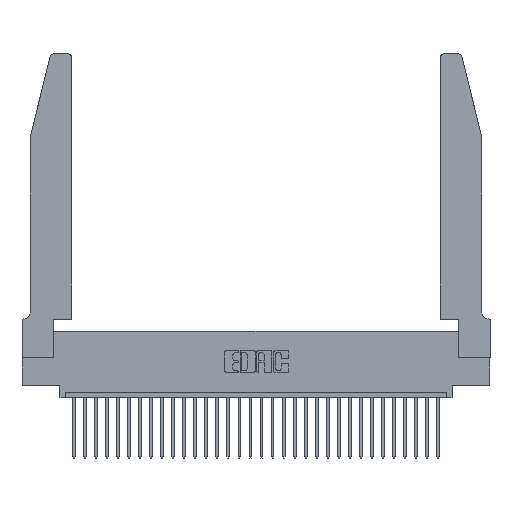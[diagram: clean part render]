
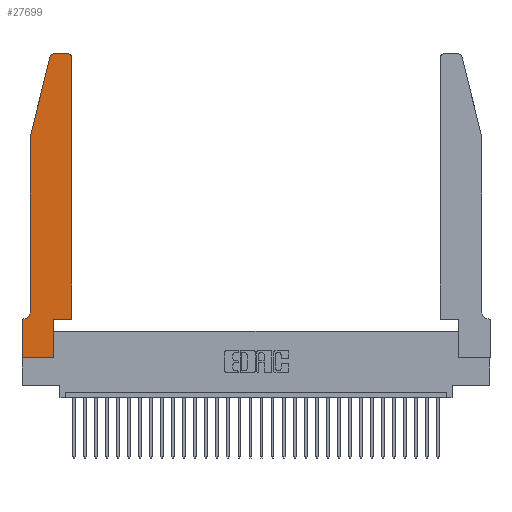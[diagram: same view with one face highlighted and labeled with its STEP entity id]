
A CAD part, top view. The second image highlights one B-rep face of the part: STEP entity #27699.
In plain terms, the highlighted planar face has unit normal (0, 0, 1).
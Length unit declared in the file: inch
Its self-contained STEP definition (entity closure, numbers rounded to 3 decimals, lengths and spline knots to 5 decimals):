
#193 = ORIENTED_EDGE ( 'NONE', *, *, #10194, .T. ) ;
#328 = CARTESIAN_POINT ( 'NONE',  ( 0.2605, 2.75, 0.37 ) ) ;
#443 = VERTEX_POINT ( 'NONE', #21732 ) ;
#835 = CARTESIAN_POINT ( 'NONE',  ( 0.0755, 2., 0.37 ) ) ;
#1008 = EDGE_CURVE ( 'NONE', #13821, #19649, #5356, .T. ) ;
#1247 = DIRECTION ( 'NONE',  ( 0., 0., 1. ) ) ;
#1374 = DIRECTION ( 'NONE',  ( 1., 0., 0. ) ) ;
#1831 = EDGE_CURVE ( 'NONE', #30188, #12874, #20572, .T. ) ;
#1934 = LINE ( 'NONE', #30293, #8049 ) ;
#1952 = CARTESIAN_POINT ( 'NONE',  ( 0.0055, 0.42, 0.37 ) ) ;
#2364 = LINE ( 'NONE', #5169, #30984 ) ;
#3104 = CARTESIAN_POINT ( 'NONE',  ( 0.0755, 0.35, 0.37 ) ) ;
#3563 = EDGE_CURVE ( 'NONE', #7966, #5126, #23149, .T. ) ;
#5004 = ORIENTED_EDGE ( 'NONE', *, *, #28620, .T. ) ;
#5009 = CARTESIAN_POINT ( 'NONE',  ( 0.0055, 0.35, 0.37 ) ) ;
#5010 = VERTEX_POINT ( 'NONE', #17199 ) ;
#5126 = VERTEX_POINT ( 'NONE', #21853 ) ;
#5169 = CARTESIAN_POINT ( 'NONE',  ( 0., 0., 0.37 ) ) ;
#5356 = CIRCLE ( 'NONE', #21744, 0.03 ) ;
#5388 = VERTEX_POINT ( 'NONE', #5009 ) ;
#5999 = EDGE_CURVE ( 'NONE', #15952, #17860, #22972, .T. ) ;
#6117 = CARTESIAN_POINT ( 'NONE',  ( 0.4505, 2.72, 0.37 ) ) ;
#6141 = DIRECTION ( 'NONE',  ( 0., 0., 1. ) ) ;
#6283 = CARTESIAN_POINT ( 'NONE',  ( 0., 0.35, 0.37 ) ) ;
#6318 = VECTOR ( 'NONE', #25117, 39.37008 ) ;
#7792 = DIRECTION ( 'NONE',  ( -1., 0., 0. ) ) ;
#7966 = VERTEX_POINT ( 'NONE', #12663 ) ;
#8049 = VECTOR ( 'NONE', #19471, 39.37008 ) ;
#8314 = DIRECTION ( 'NONE',  ( 0., 1., 0. ) ) ;
#9087 = CARTESIAN_POINT ( 'NONE',  ( 0.0755, 0.42, 0.37 ) ) ;
#9263 = DIRECTION ( 'NONE',  ( 1., 0., 0. ) ) ;
#10145 = CARTESIAN_POINT ( 'NONE',  ( 0.2865, 0.35, 0.37 ) ) ;
#10194 = EDGE_CURVE ( 'NONE', #5388, #23046, #20804, .T. ) ;
#10940 = ORIENTED_EDGE ( 'NONE', *, *, #12005, .T. ) ;
#11114 = DIRECTION ( 'NONE',  ( 0., -1., 0. ) ) ;
#11465 = VECTOR ( 'NONE', #12480, 39.37008 ) ;
#11828 = DIRECTION ( 'NONE',  ( 0., 0., 1. ) ) ;
#12005 = EDGE_CURVE ( 'NONE', #17860, #13821, #12695, .T. ) ;
#12480 = DIRECTION ( 'NONE',  ( 1., 0., 0. ) ) ;
#12663 = CARTESIAN_POINT ( 'NONE',  ( 0.2865, 0.35, 0.37 ) ) ;
#12695 = LINE ( 'NONE', #328, #15411 ) ;
#12874 = VERTEX_POINT ( 'NONE', #9087 ) ;
#13300 = DIRECTION ( 'NONE',  ( 1., 0., 0. ) ) ;
#13702 = AXIS2_PLACEMENT_3D ( 'NONE', #6283, #1247, #18309 ) ;
#13821 = VERTEX_POINT ( 'NONE', #20602 ) ;
#14493 = ORIENTED_EDGE ( 'NONE', *, *, #25346, .T. ) ;
#14534 = LINE ( 'NONE', #27191, #11465 ) ;
#14662 = ORIENTED_EDGE ( 'NONE', *, *, #5999, .T. ) ;
#15411 = VECTOR ( 'NONE', #7792, 39.37008 ) ;
#15952 = VERTEX_POINT ( 'NONE', #6117 ) ;
#16477 = ORIENTED_EDGE ( 'NONE', *, *, #1008, .T. ) ;
#16829 = CARTESIAN_POINT ( 'NONE',  ( 0., 0.35, 0.37 ) ) ;
#17199 = CARTESIAN_POINT ( 'NONE',  ( 0., 0., 0.37 ) ) ;
#17707 = EDGE_CURVE ( 'NONE', #12874, #5388, #19935, .T. ) ;
#17860 = VERTEX_POINT ( 'NONE', #22608 ) ;
#17881 = ORIENTED_EDGE ( 'NONE', *, *, #25111, .T. ) ;
#17967 = CARTESIAN_POINT ( 'NONE',  ( 0.4205, 2.72, 0.37 ) ) ;
#18288 = ORIENTED_EDGE ( 'NONE', *, *, #1831, .T. ) ;
#18309 = DIRECTION ( 'NONE',  ( 1., 0., 0. ) ) ;
#19471 = DIRECTION ( 'NONE',  ( 0., 1., 0. ) ) ;
#19545 = EDGE_LOOP ( 'NONE', ( #10940, #16477, #30060, #18288, #30279, #193, #24471, #17881, #14493, #23701, #5004, #14662 ) ) ;
#19649 = VERTEX_POINT ( 'NONE', #25116 ) ;
#19704 = VECTOR ( 'NONE', #29470, 39.37008 ) ;
#19935 = CIRCLE ( 'NONE', #29389, 0.07 ) ;
#20240 = CARTESIAN_POINT ( 'NONE',  ( 0.0755, 2., 0.37 ) ) ;
#20572 = LINE ( 'NONE', #20240, #29701 ) ;
#20602 = CARTESIAN_POINT ( 'NONE',  ( 0.284, 2.75, 0.37 ) ) ;
#20804 = LINE ( 'NONE', #3104, #6318 ) ;
#21574 = VECTOR ( 'NONE', #8314, 39.37008 ) ;
#21609 = CARTESIAN_POINT ( 'NONE',  ( 0.284, 2.72, 0.37 ) ) ;
#21732 = CARTESIAN_POINT ( 'NONE',  ( 0.2865, 0., 0.37 ) ) ;
#21744 = AXIS2_PLACEMENT_3D ( 'NONE', #21609, #11828, #9263 ) ;
#21853 = CARTESIAN_POINT ( 'NONE',  ( 0.4505, 0.35, 0.37 ) ) ;
#22248 = DIRECTION ( 'NONE',  ( 0., -1., 0. ) ) ;
#22608 = CARTESIAN_POINT ( 'NONE',  ( 0.4205, 2.75, 0.37 ) ) ;
#22972 = CIRCLE ( 'NONE', #30607, 0.03 ) ;
#23046 = VERTEX_POINT ( 'NONE', #16829 ) ;
#23149 = LINE ( 'NONE', #28476, #23526 ) ;
#23526 = VECTOR ( 'NONE', #1374, 39.37008 ) ;
#23585 = PLANE ( 'NONE',  #13702 ) ;
#23701 = ORIENTED_EDGE ( 'NONE', *, *, #3563, .T. ) ;
#23745 = EDGE_CURVE ( 'NONE', #19649, #30188, #25466, .T. ) ;
#23760 = DIRECTION ( 'NONE',  ( -1., 0., 0. ) ) ;
#24471 = ORIENTED_EDGE ( 'NONE', *, *, #27969, .T. ) ;
#25111 = EDGE_CURVE ( 'NONE', #5010, #443, #14534, .T. ) ;
#25116 = CARTESIAN_POINT ( 'NONE',  ( 0.25487, 2.72718, 0.37 ) ) ;
#25117 = DIRECTION ( 'NONE',  ( -1., 0., 0. ) ) ;
#25346 = EDGE_CURVE ( 'NONE', #443, #7966, #31505, .T. ) ;
#25466 = LINE ( 'NONE', #835, #19704 ) ;
#27191 = CARTESIAN_POINT ( 'NONE',  ( 0., 0., 0.37 ) ) ;
#27699 = ADVANCED_FACE ( 'NONE', ( #31013 ), #23585, .T. ) ;
#27969 = EDGE_CURVE ( 'NONE', #23046, #5010, #2364, .T. ) ;
#28476 = CARTESIAN_POINT ( 'NONE',  ( 0.4505, 0.35, 0.37 ) ) ;
#28620 = EDGE_CURVE ( 'NONE', #5126, #15952, #1934, .T. ) ;
#29389 = AXIS2_PLACEMENT_3D ( 'NONE', #1952, #31071, #23760 ) ;
#29470 = DIRECTION ( 'NONE',  ( -0.239, -0.971, 0. ) ) ;
#29701 = VECTOR ( 'NONE', #11114, 39.37008 ) ;
#30060 = ORIENTED_EDGE ( 'NONE', *, *, #23745, .T. ) ;
#30188 = VERTEX_POINT ( 'NONE', #30981 ) ;
#30279 = ORIENTED_EDGE ( 'NONE', *, *, #17707, .T. ) ;
#30293 = CARTESIAN_POINT ( 'NONE',  ( 0.4505, 0.35, 0.37 ) ) ;
#30607 = AXIS2_PLACEMENT_3D ( 'NONE', #17967, #6141, #13300 ) ;
#30981 = CARTESIAN_POINT ( 'NONE',  ( 0.0755, 2., 0.37 ) ) ;
#30984 = VECTOR ( 'NONE', #22248, 39.37008 ) ;
#31013 = FACE_OUTER_BOUND ( 'NONE', #19545, .T. ) ;
#31071 = DIRECTION ( 'NONE',  ( 0., 0., -1. ) ) ;
#31505 = LINE ( 'NONE', #10145, #21574 ) ;
